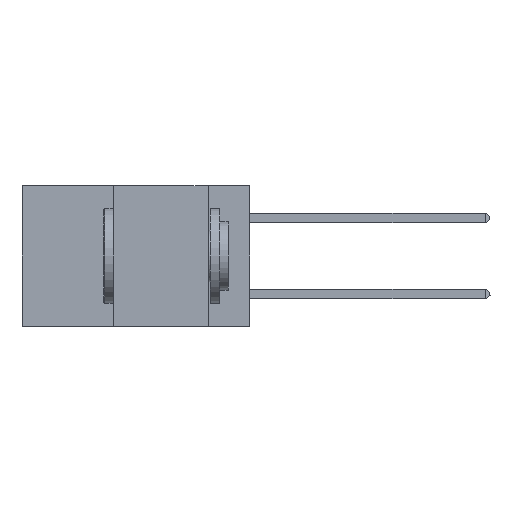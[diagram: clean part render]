
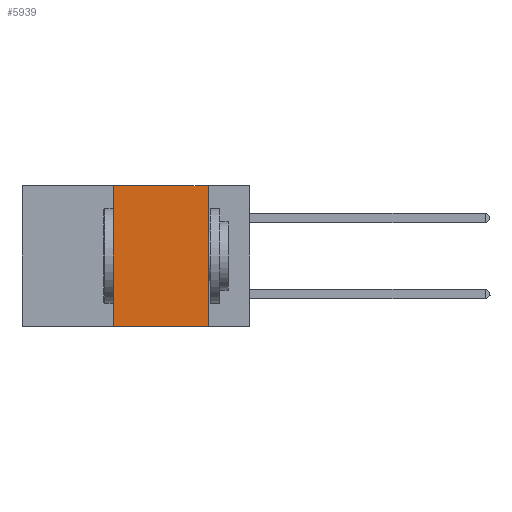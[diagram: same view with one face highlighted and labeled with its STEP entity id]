
A CAD part, left-side view. The second image highlights one B-rep face of the part: STEP entity #5939.
In plain terms, the highlighted planar face has unit normal (-1, 0, 0).
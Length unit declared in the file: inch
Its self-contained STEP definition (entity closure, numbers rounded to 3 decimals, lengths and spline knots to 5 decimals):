
#128 = DIRECTION ( 'NONE',  ( 0., 0., -1. ) ) ;
#186 = DIRECTION ( 'NONE',  ( 1., 0., 0. ) ) ;
#483 = EDGE_CURVE ( 'NONE', #5773, #7384, #1779, .T. ) ;
#495 = ORIENTED_EDGE ( 'NONE', *, *, #8918, .F. ) ;
#544 = CARTESIAN_POINT ( 'NONE',  ( 0., 0.36, 0. ) ) ;
#1022 = PLANE ( 'NONE',  #9039 ) ;
#1494 = VERTEX_POINT ( 'NONE', #544 ) ;
#1628 = VECTOR ( 'NONE', #3213, 39.37008 ) ;
#1779 = LINE ( 'NONE', #9706, #7349 ) ;
#1870 = CARTESIAN_POINT ( 'NONE',  ( 0., 0.6, 0. ) ) ;
#2385 = ORIENTED_EDGE ( 'NONE', *, *, #483, .F. ) ;
#2482 = LINE ( 'NONE', #5699, #6527 ) ;
#2896 = ORIENTED_EDGE ( 'NONE', *, *, #9379, .F. ) ;
#3213 = DIRECTION ( 'NONE',  ( 0., -1., 0. ) ) ;
#4493 = VERTEX_POINT ( 'NONE', #7019 ) ;
#4771 = CARTESIAN_POINT ( 'NONE',  ( 0., 0.11, 0. ) ) ;
#5535 = DIRECTION ( 'NONE',  ( 0., 0., 1. ) ) ;
#5546 = CARTESIAN_POINT ( 'NONE',  ( 0., 0.11, -0.37 ) ) ;
#5568 = VECTOR ( 'NONE', #8623, 39.37008 ) ;
#5699 = CARTESIAN_POINT ( 'NONE',  ( 0., 0.36, 0. ) ) ;
#5711 = LINE ( 'NONE', #7673, #1628 ) ;
#5773 = VERTEX_POINT ( 'NONE', #4771 ) ;
#5939 = ADVANCED_FACE ( 'NONE', ( #8985 ), #1022, .F. ) ;
#6527 = VECTOR ( 'NONE', #5535, 39.37008 ) ;
#6578 = EDGE_CURVE ( 'NONE', #4493, #7384, #5711, .T. ) ;
#7019 = CARTESIAN_POINT ( 'NONE',  ( 0., 0.36, -0.37 ) ) ;
#7349 = VECTOR ( 'NONE', #9551, 39.37008 ) ;
#7384 = VERTEX_POINT ( 'NONE', #5546 ) ;
#7673 = CARTESIAN_POINT ( 'NONE',  ( 0., 0.6, -0.37 ) ) ;
#7754 = LINE ( 'NONE', #8563, #5568 ) ;
#8563 = CARTESIAN_POINT ( 'NONE',  ( 0., 0.6, 0. ) ) ;
#8592 = ORIENTED_EDGE ( 'NONE', *, *, #6578, .T. ) ;
#8623 = DIRECTION ( 'NONE',  ( 0., -1., 0. ) ) ;
#8787 = EDGE_LOOP ( 'NONE', ( #2385, #495, #2896, #8592 ) ) ;
#8918 = EDGE_CURVE ( 'NONE', #1494, #5773, #7754, .T. ) ;
#8985 = FACE_OUTER_BOUND ( 'NONE', #8787, .T. ) ;
#9039 = AXIS2_PLACEMENT_3D ( 'NONE', #1870, #186, #128 ) ;
#9379 = EDGE_CURVE ( 'NONE', #4493, #1494, #2482, .T. ) ;
#9551 = DIRECTION ( 'NONE',  ( 0., 0., -1. ) ) ;
#9706 = CARTESIAN_POINT ( 'NONE',  ( 0., 0.11, 0. ) ) ;
